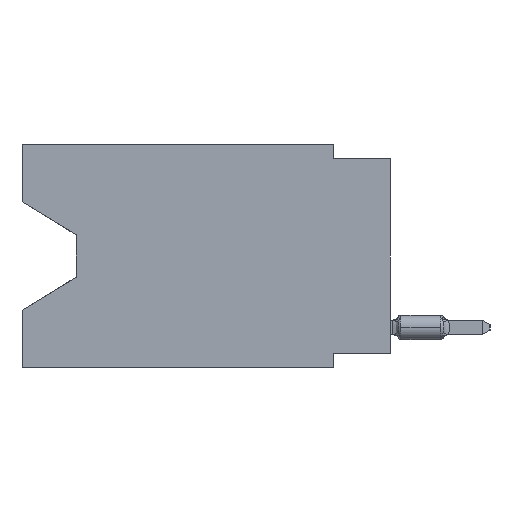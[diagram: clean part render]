
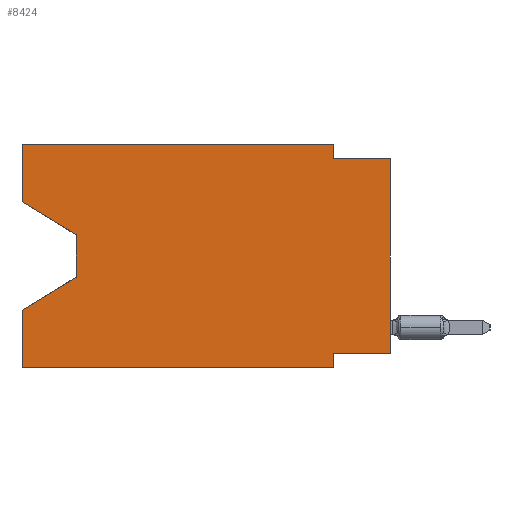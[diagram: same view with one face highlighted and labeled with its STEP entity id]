
A CAD part, left-side view. The second image highlights one B-rep face of the part: STEP entity #8424.
In plain terms, the highlighted planar face has unit normal (-1, 0, 0).
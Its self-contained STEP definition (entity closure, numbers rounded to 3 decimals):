
#470 = DIRECTION ( 'NONE',  ( 0., 0., -1. ) ) ;
#550 = ORIENTED_EDGE ( 'NONE', *, *, #22086, .F. ) ;
#1138 = CARTESIAN_POINT ( 'NONE',  ( 0., 2.54, -0.635 ) ) ;
#1718 = EDGE_CURVE ( 'NONE', #20525, #72269, #25438, .T. ) ;
#3339 = VERTEX_POINT ( 'NONE', #17902 ) ;
#4061 = ORIENTED_EDGE ( 'NONE', *, *, #43676, .F. ) ;
#4530 = LINE ( 'NONE', #73384, #17966 ) ;
#5371 = VECTOR ( 'NONE', #63592, 1000. ) ;
#5519 = ORIENTED_EDGE ( 'NONE', *, *, #23953, .T. ) ;
#7654 = CARTESIAN_POINT ( 'NONE',  ( 0., 0., -9.271 ) ) ;
#7805 = LINE ( 'NONE', #30744, #31931 ) ;
#8233 = LINE ( 'NONE', #25507, #12263 ) ;
#8424 = ADVANCED_FACE ( 'NONE', ( #28325 ), #74258, .F. ) ;
#9339 = DIRECTION ( 'NONE',  ( 0., 0., -1. ) ) ;
#9574 = VERTEX_POINT ( 'NONE', #23470 ) ;
#10598 = CARTESIAN_POINT ( 'NONE',  ( 0., 16.383, -7.36 ) ) ;
#11582 = VERTEX_POINT ( 'NONE', #31436 ) ;
#12040 = CARTESIAN_POINT ( 'NONE',  ( 0., 2.54, -9.906 ) ) ;
#12263 = VECTOR ( 'NONE', #9339, 1000. ) ;
#13189 = CARTESIAN_POINT ( 'NONE',  ( 0., 13.97, -4.013 ) ) ;
#14308 = CARTESIAN_POINT ( 'NONE',  ( 0., 13.97, -4.013 ) ) ;
#14804 = VECTOR ( 'NONE', #64452, 1000. ) ;
#15323 = VECTOR ( 'NONE', #38588, 1000. ) ;
#16447 = ORIENTED_EDGE ( 'NONE', *, *, #30233, .T. ) ;
#16915 = DIRECTION ( 'NONE',  ( 0., 0., -1. ) ) ;
#17902 = CARTESIAN_POINT ( 'NONE',  ( 0., 2.54, 0. ) ) ;
#17966 = VECTOR ( 'NONE', #67739, 1000. ) ;
#18946 = VERTEX_POINT ( 'NONE', #1138 ) ;
#19624 = EDGE_LOOP ( 'NONE', ( #21680, #16447, #24723, #22936, #5519, #550, #4061, #66569, #61256, #55196, #35317, #23617 ) ) ;
#19768 = EDGE_CURVE ( 'NONE', #54162, #28456, #70118, .T. ) ;
#20525 = VERTEX_POINT ( 'NONE', #44728 ) ;
#21169 = EDGE_CURVE ( 'NONE', #11582, #28456, #40264, .T. ) ;
#21680 = ORIENTED_EDGE ( 'NONE', *, *, #23812, .T. ) ;
#22086 = EDGE_CURVE ( 'NONE', #47502, #9574, #39524, .T. ) ;
#22936 = ORIENTED_EDGE ( 'NONE', *, *, #21169, .F. ) ;
#23470 = CARTESIAN_POINT ( 'NONE',  ( 0., 2.54, -9.906 ) ) ;
#23617 = ORIENTED_EDGE ( 'NONE', *, *, #1718, .F. ) ;
#23812 = EDGE_CURVE ( 'NONE', #20525, #31456, #63508, .T. ) ;
#23953 = EDGE_CURVE ( 'NONE', #11582, #9574, #7805, .T. ) ;
#24244 = VECTOR ( 'NONE', #60816, 1000. ) ;
#24723 = ORIENTED_EDGE ( 'NONE', *, *, #19768, .T. ) ;
#25438 = LINE ( 'NONE', #37846, #24244 ) ;
#25507 = CARTESIAN_POINT ( 'NONE',  ( 0., 2.54, 0. ) ) ;
#26643 = VECTOR ( 'NONE', #70516, 1000. ) ;
#28325 = FACE_OUTER_BOUND ( 'NONE', #19624, .T. ) ;
#28456 = VERTEX_POINT ( 'NONE', #10598 ) ;
#29269 = CARTESIAN_POINT ( 'NONE',  ( 0., 16.383, -2.546 ) ) ;
#30233 = EDGE_CURVE ( 'NONE', #31456, #54162, #43267, .T. ) ;
#30744 = CARTESIAN_POINT ( 'NONE',  ( 0., 16.383, -9.906 ) ) ;
#31436 = CARTESIAN_POINT ( 'NONE',  ( 0., 16.383, -9.906 ) ) ;
#31456 = VERTEX_POINT ( 'NONE', #14308 ) ;
#31630 = EDGE_CURVE ( 'NONE', #72269, #3339, #4530, .T. ) ;
#31931 = VECTOR ( 'NONE', #60082, 1000. ) ;
#32127 = DIRECTION ( 'NONE',  ( 0., 0., 1. ) ) ;
#34345 = DIRECTION ( 'NONE',  ( 1., 0., 0. ) ) ;
#35317 = ORIENTED_EDGE ( 'NONE', *, *, #31630, .F. ) ;
#35486 = VECTOR ( 'NONE', #16915, 1000. ) ;
#37707 = LINE ( 'NONE', #7654, #26643 ) ;
#37846 = CARTESIAN_POINT ( 'NONE',  ( 0., 16.383, 0. ) ) ;
#38491 = VECTOR ( 'NONE', #64747, 1000. ) ;
#38588 = DIRECTION ( 'NONE',  ( 0., -1., 0. ) ) ;
#39524 = LINE ( 'NONE', #12040, #35486 ) ;
#39694 = LINE ( 'NONE', #45339, #15323 ) ;
#40091 = VERTEX_POINT ( 'NONE', #65035 ) ;
#40264 = LINE ( 'NONE', #68889, #5371 ) ;
#42804 = VECTOR ( 'NONE', #32127, 1000. ) ;
#43267 = LINE ( 'NONE', #13189, #38491 ) ;
#43676 = EDGE_CURVE ( 'NONE', #71030, #47502, #37707, .T. ) ;
#44728 = CARTESIAN_POINT ( 'NONE',  ( 0., 16.383, -2.546 ) ) ;
#45339 = CARTESIAN_POINT ( 'NONE',  ( 0., 0., -0.635 ) ) ;
#47502 = VERTEX_POINT ( 'NONE', #50163 ) ;
#47662 = AXIS2_PLACEMENT_3D ( 'NONE', #67866, #34345, #470 ) ;
#50163 = CARTESIAN_POINT ( 'NONE',  ( 0., 2.54, -9.271 ) ) ;
#50313 = EDGE_CURVE ( 'NONE', #18946, #40091, #39694, .T. ) ;
#50582 = CARTESIAN_POINT ( 'NONE',  ( 0., 16.383, 0. ) ) ;
#51462 = CARTESIAN_POINT ( 'NONE',  ( 0., 0., -9.271 ) ) ;
#52215 = DIRECTION ( 'NONE',  ( 0., -0.855, -0.519 ) ) ;
#54162 = VERTEX_POINT ( 'NONE', #55112 ) ;
#55112 = CARTESIAN_POINT ( 'NONE',  ( 0., 13.97, -5.893 ) ) ;
#55196 = ORIENTED_EDGE ( 'NONE', *, *, #69774, .F. ) ;
#55819 = CARTESIAN_POINT ( 'NONE',  ( 0., 0., 0. ) ) ;
#60082 = DIRECTION ( 'NONE',  ( 0., -1., 0. ) ) ;
#60816 = DIRECTION ( 'NONE',  ( 0., 0., 1. ) ) ;
#61256 = ORIENTED_EDGE ( 'NONE', *, *, #50313, .F. ) ;
#63344 = CARTESIAN_POINT ( 'NONE',  ( 0., 13.97, -5.893 ) ) ;
#63508 = LINE ( 'NONE', #29269, #71595 ) ;
#63592 = DIRECTION ( 'NONE',  ( 0., 0., 1. ) ) ;
#63996 = EDGE_CURVE ( 'NONE', #71030, #40091, #72035, .T. ) ;
#64452 = DIRECTION ( 'NONE',  ( 0., 0.855, -0.519 ) ) ;
#64747 = DIRECTION ( 'NONE',  ( 0., 0., -1. ) ) ;
#65035 = CARTESIAN_POINT ( 'NONE',  ( 0., 0., -0.635 ) ) ;
#66569 = ORIENTED_EDGE ( 'NONE', *, *, #63996, .T. ) ;
#67739 = DIRECTION ( 'NONE',  ( 0., -1., 0. ) ) ;
#67866 = CARTESIAN_POINT ( 'NONE',  ( 0., 16.383, 0. ) ) ;
#68889 = CARTESIAN_POINT ( 'NONE',  ( 0., 16.383, 0. ) ) ;
#69774 = EDGE_CURVE ( 'NONE', #3339, #18946, #8233, .T. ) ;
#70118 = LINE ( 'NONE', #63344, #14804 ) ;
#70516 = DIRECTION ( 'NONE',  ( 0., 1., 0. ) ) ;
#71030 = VERTEX_POINT ( 'NONE', #51462 ) ;
#71595 = VECTOR ( 'NONE', #52215, 1000. ) ;
#72035 = LINE ( 'NONE', #55819, #42804 ) ;
#72269 = VERTEX_POINT ( 'NONE', #50582 ) ;
#73384 = CARTESIAN_POINT ( 'NONE',  ( 0., 16.383, 0. ) ) ;
#74258 = PLANE ( 'NONE',  #47662 ) ;
